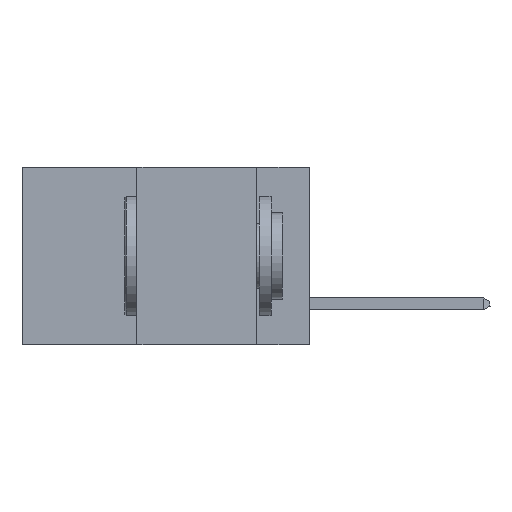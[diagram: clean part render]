
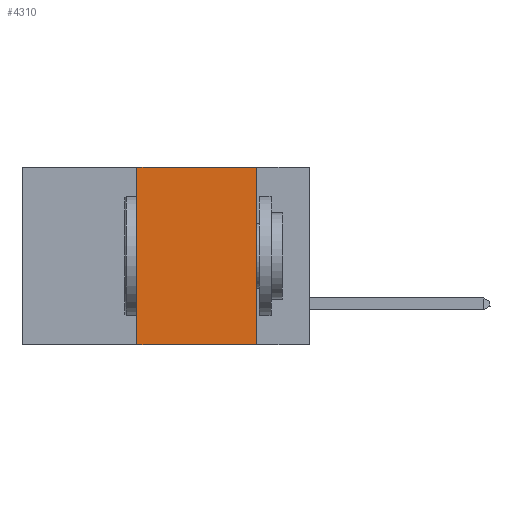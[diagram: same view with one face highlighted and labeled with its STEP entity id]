
A CAD part, left-side view. The second image highlights one B-rep face of the part: STEP entity #4310.
In plain terms, the highlighted planar face has unit normal (-1, 0, 0).
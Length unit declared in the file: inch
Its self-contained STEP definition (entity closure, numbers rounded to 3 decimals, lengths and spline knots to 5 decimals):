
#837 = ORIENTED_EDGE ( 'NONE', *, *, #9937, .F. ) ;
#1507 = VECTOR ( 'NONE', #6428, 39.37008 ) ;
#4135 = AXIS2_PLACEMENT_3D ( 'NONE', #13770, #38846, #6168 ) ;
#4163 = DIRECTION ( 'NONE',  ( 0., -1., 0. ) ) ;
#4310 = ADVANCED_FACE ( 'NONE', ( #19916 ), #42861, .F. ) ;
#5090 = ORIENTED_EDGE ( 'NONE', *, *, #37661, .T. ) ;
#5865 = CARTESIAN_POINT ( 'NONE',  ( 0., 0.11, -0.37 ) ) ;
#6168 = DIRECTION ( 'NONE',  ( 0., 0., -1. ) ) ;
#6428 = DIRECTION ( 'NONE',  ( 0., 0., 1. ) ) ;
#7540 = ORIENTED_EDGE ( 'NONE', *, *, #21366, .F. ) ;
#7717 = LINE ( 'NONE', #16573, #13511 ) ;
#9609 = VECTOR ( 'NONE', #23094, 39.37008 ) ;
#9937 = EDGE_CURVE ( 'NONE', #31604, #28385, #10932, .T. ) ;
#10932 = LINE ( 'NONE', #23241, #1507 ) ;
#12641 = CARTESIAN_POINT ( 'NONE',  ( 0., 0.11, 0. ) ) ;
#13511 = VECTOR ( 'NONE', #34090, 39.37008 ) ;
#13770 = CARTESIAN_POINT ( 'NONE',  ( 0., 0.6, 0. ) ) ;
#14686 = CARTESIAN_POINT ( 'NONE',  ( 0., 0.36, -0.37 ) ) ;
#16573 = CARTESIAN_POINT ( 'NONE',  ( 0., 0.6, -0.37 ) ) ;
#16596 = EDGE_CURVE ( 'NONE', #28385, #21040, #28796, .T. ) ;
#19592 = LINE ( 'NONE', #12641, #9609 ) ;
#19916 = FACE_OUTER_BOUND ( 'NONE', #32611, .T. ) ;
#20160 = ORIENTED_EDGE ( 'NONE', *, *, #16596, .F. ) ;
#21040 = VERTEX_POINT ( 'NONE', #37217 ) ;
#21366 = EDGE_CURVE ( 'NONE', #21040, #25329, #19592, .T. ) ;
#23094 = DIRECTION ( 'NONE',  ( 0., 0., -1. ) ) ;
#23241 = CARTESIAN_POINT ( 'NONE',  ( 0., 0.36, 0. ) ) ;
#25329 = VERTEX_POINT ( 'NONE', #5865 ) ;
#28385 = VERTEX_POINT ( 'NONE', #43185 ) ;
#28796 = LINE ( 'NONE', #34113, #38127 ) ;
#31604 = VERTEX_POINT ( 'NONE', #14686 ) ;
#32611 = EDGE_LOOP ( 'NONE', ( #7540, #20160, #837, #5090 ) ) ;
#34090 = DIRECTION ( 'NONE',  ( 0., -1., 0. ) ) ;
#34113 = CARTESIAN_POINT ( 'NONE',  ( 0., 0.6, 0. ) ) ;
#37217 = CARTESIAN_POINT ( 'NONE',  ( 0., 0.11, 0. ) ) ;
#37661 = EDGE_CURVE ( 'NONE', #31604, #25329, #7717, .T. ) ;
#38127 = VECTOR ( 'NONE', #4163, 39.37008 ) ;
#38846 = DIRECTION ( 'NONE',  ( 1., 0., 0. ) ) ;
#42861 = PLANE ( 'NONE',  #4135 ) ;
#43185 = CARTESIAN_POINT ( 'NONE',  ( 0., 0.36, 0. ) ) ;
